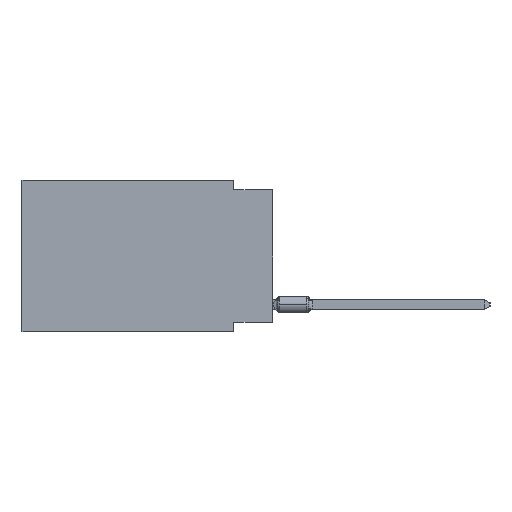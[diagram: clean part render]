
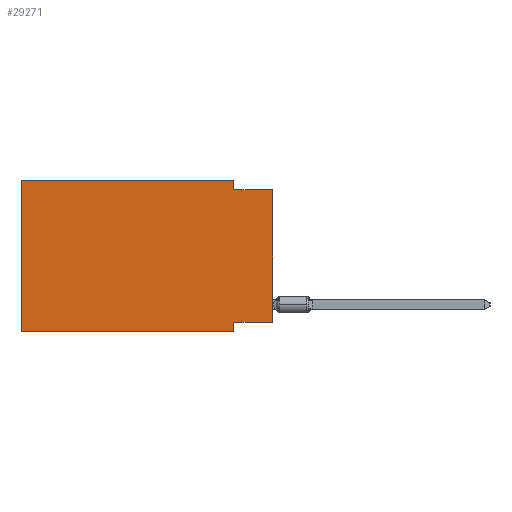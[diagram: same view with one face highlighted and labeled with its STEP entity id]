
A CAD part, left-side view. The second image highlights one B-rep face of the part: STEP entity #29271.
In plain terms, the highlighted planar face has unit normal (-1, 0, 0).
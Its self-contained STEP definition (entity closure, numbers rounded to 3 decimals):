
#621 = VERTEX_POINT ( 'NONE', #3761 ) ;
#3580 = LINE ( 'NONE', #49741, #51725 ) ;
#3608 = DIRECTION ( 'NONE',  ( 0., 0., -1. ) ) ;
#3761 = CARTESIAN_POINT ( 'NONE',  ( 0., 0., -0.635 ) ) ;
#4552 = VERTEX_POINT ( 'NONE', #50135 ) ;
#4967 = DIRECTION ( 'NONE',  ( 0., 0., 1. ) ) ;
#5720 = EDGE_CURVE ( 'NONE', #66255, #26795, #33811, .T. ) ;
#6612 = CARTESIAN_POINT ( 'NONE',  ( 0., 16.383, -9.906 ) ) ;
#13129 = ORIENTED_EDGE ( 'NONE', *, *, #5720, .F. ) ;
#13428 = DIRECTION ( 'NONE',  ( 0., -1., 0. ) ) ;
#13666 = CARTESIAN_POINT ( 'NONE',  ( 0., 16.383, 0. ) ) ;
#13991 = ORIENTED_EDGE ( 'NONE', *, *, #38077, .T. ) ;
#14253 = DIRECTION ( 'NONE',  ( 1., 0., 0. ) ) ;
#14498 = EDGE_LOOP ( 'NONE', ( #13991, #29325, #56363, #45196, #13129, #28751, #34160, #40404 ) ) ;
#14597 = FACE_OUTER_BOUND ( 'NONE', #14498, .T. ) ;
#17605 = VECTOR ( 'NONE', #42676, 1000. ) ;
#18066 = VECTOR ( 'NONE', #3608, 1000. ) ;
#21344 = CARTESIAN_POINT ( 'NONE',  ( 0., 2.54, 0. ) ) ;
#21928 = VERTEX_POINT ( 'NONE', #43696 ) ;
#22468 = CARTESIAN_POINT ( 'NONE',  ( 0., 2.54, -9.906 ) ) ;
#26795 = VERTEX_POINT ( 'NONE', #58971 ) ;
#26909 = LINE ( 'NONE', #22468, #39554 ) ;
#26979 = EDGE_CURVE ( 'NONE', #21928, #621, #3580, .T. ) ;
#27373 = VECTOR ( 'NONE', #39956, 1000. ) ;
#27975 = AXIS2_PLACEMENT_3D ( 'NONE', #29969, #14253, #46013 ) ;
#28246 = CARTESIAN_POINT ( 'NONE',  ( 0., 2.54, 0. ) ) ;
#28751 = ORIENTED_EDGE ( 'NONE', *, *, #67164, .T. ) ;
#29271 = ADVANCED_FACE ( 'NONE', ( #14597 ), #45663, .F. ) ;
#29325 = ORIENTED_EDGE ( 'NONE', *, *, #26979, .F. ) ;
#29969 = CARTESIAN_POINT ( 'NONE',  ( 0., 16.383, 0. ) ) ;
#30392 = EDGE_CURVE ( 'NONE', #26795, #67424, #39385, .T. ) ;
#33652 = DIRECTION ( 'NONE',  ( 0., -1., 0. ) ) ;
#33811 = LINE ( 'NONE', #13666, #27373 ) ;
#34160 = ORIENTED_EDGE ( 'NONE', *, *, #39795, .F. ) ;
#36180 = EDGE_CURVE ( 'NONE', #44013, #4552, #60034, .T. ) ;
#37195 = CARTESIAN_POINT ( 'NONE',  ( 0., 16.383, -9.906 ) ) ;
#38077 = EDGE_CURVE ( 'NONE', #44013, #621, #45635, .T. ) ;
#39385 = LINE ( 'NONE', #60220, #57739 ) ;
#39554 = VECTOR ( 'NONE', #63465, 1000. ) ;
#39795 = EDGE_CURVE ( 'NONE', #4552, #66581, #26909, .T. ) ;
#39956 = DIRECTION ( 'NONE',  ( 0., 0., 1. ) ) ;
#40404 = ORIENTED_EDGE ( 'NONE', *, *, #36180, .F. ) ;
#41749 = CARTESIAN_POINT ( 'NONE',  ( 0., 2.54, -9.906 ) ) ;
#42676 = DIRECTION ( 'NONE',  ( 0., -1., 0. ) ) ;
#43290 = CARTESIAN_POINT ( 'NONE',  ( 0., 0., -9.271 ) ) ;
#43696 = CARTESIAN_POINT ( 'NONE',  ( 0., 2.54, -0.635 ) ) ;
#44013 = VERTEX_POINT ( 'NONE', #43290 ) ;
#44033 = EDGE_CURVE ( 'NONE', #67424, #21928, #54886, .T. ) ;
#45196 = ORIENTED_EDGE ( 'NONE', *, *, #30392, .F. ) ;
#45635 = LINE ( 'NONE', #66151, #63400 ) ;
#45663 = PLANE ( 'NONE',  #27975 ) ;
#46013 = DIRECTION ( 'NONE',  ( 0., 0., -1. ) ) ;
#48212 = VECTOR ( 'NONE', #60370, 1000. ) ;
#48467 = LINE ( 'NONE', #37195, #17605 ) ;
#49741 = CARTESIAN_POINT ( 'NONE',  ( 0., 0., -0.635 ) ) ;
#50135 = CARTESIAN_POINT ( 'NONE',  ( 0., 2.54, -9.271 ) ) ;
#51725 = VECTOR ( 'NONE', #33652, 1000. ) ;
#54886 = LINE ( 'NONE', #28246, #18066 ) ;
#56363 = ORIENTED_EDGE ( 'NONE', *, *, #44033, .F. ) ;
#57739 = VECTOR ( 'NONE', #13428, 1000. ) ;
#58971 = CARTESIAN_POINT ( 'NONE',  ( 0., 16.383, 0. ) ) ;
#60034 = LINE ( 'NONE', #65500, #48212 ) ;
#60220 = CARTESIAN_POINT ( 'NONE',  ( 0., 16.383, 0. ) ) ;
#60370 = DIRECTION ( 'NONE',  ( 0., 1., 0. ) ) ;
#63400 = VECTOR ( 'NONE', #4967, 1000. ) ;
#63465 = DIRECTION ( 'NONE',  ( 0., 0., -1. ) ) ;
#65500 = CARTESIAN_POINT ( 'NONE',  ( 0., 0., -9.271 ) ) ;
#66151 = CARTESIAN_POINT ( 'NONE',  ( 0., 0., 0. ) ) ;
#66255 = VERTEX_POINT ( 'NONE', #6612 ) ;
#66581 = VERTEX_POINT ( 'NONE', #41749 ) ;
#67164 = EDGE_CURVE ( 'NONE', #66255, #66581, #48467, .T. ) ;
#67424 = VERTEX_POINT ( 'NONE', #21344 ) ;
